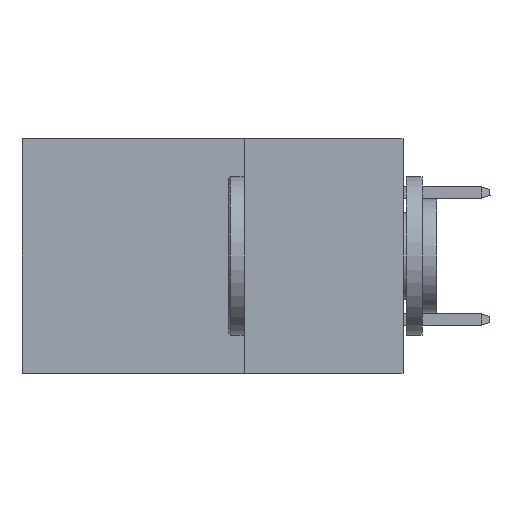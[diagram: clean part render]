
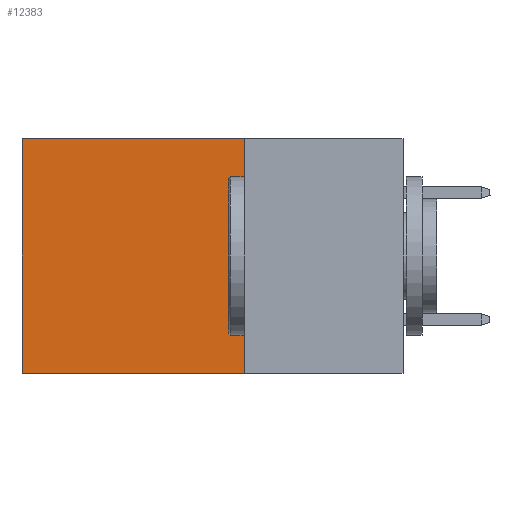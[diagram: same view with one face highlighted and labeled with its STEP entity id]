
A CAD part, left-side view. The second image highlights one B-rep face of the part: STEP entity #12383.
In plain terms, the highlighted planar face has unit normal (-1, 0, 0).
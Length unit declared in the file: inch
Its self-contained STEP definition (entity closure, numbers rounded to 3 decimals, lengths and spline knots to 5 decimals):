
#3955 = VERTEX_POINT ( 'NONE', #8767 ) ;
#5047 = DIRECTION ( 'NONE',  ( 0., 1., 0. ) ) ;
#6533 = ORIENTED_EDGE ( 'NONE', *, *, #20323, .T. ) ;
#8109 = DIRECTION ( 'NONE',  ( 0., 1., 0. ) ) ;
#8767 = CARTESIAN_POINT ( 'NONE',  ( 0.2875, 0.25, -0.37 ) ) ;
#9014 = CARTESIAN_POINT ( 'NONE',  ( 0.2875, 0.25, 0. ) ) ;
#9194 = ORIENTED_EDGE ( 'NONE', *, *, #35555, .F. ) ;
#11284 = CARTESIAN_POINT ( 'NONE',  ( 0.2875, 0.25, 0. ) ) ;
#11391 = VERTEX_POINT ( 'NONE', #26016 ) ;
#12294 = DIRECTION ( 'NONE',  ( 0., 0., -1. ) ) ;
#12383 = ADVANCED_FACE ( 'NONE', ( #35965 ), #30288, .F. ) ;
#14597 = CARTESIAN_POINT ( 'NONE',  ( 0.2875, 0.25, 0. ) ) ;
#16473 = EDGE_CURVE ( 'NONE', #29625, #3955, #30131, .T. ) ;
#16636 = CARTESIAN_POINT ( 'NONE',  ( 0.2875, 0.25, -0.37 ) ) ;
#20323 = EDGE_CURVE ( 'NONE', #29625, #11391, #28796, .T. ) ;
#21387 = CARTESIAN_POINT ( 'NONE',  ( 0.2875, 0.25, 0. ) ) ;
#22755 = EDGE_CURVE ( 'NONE', #11391, #36157, #24646, .T. ) ;
#23170 = LINE ( 'NONE', #16636, #23257 ) ;
#23257 = VECTOR ( 'NONE', #5047, 39.37008 ) ;
#24646 = LINE ( 'NONE', #25030, #35932 ) ;
#25019 = CARTESIAN_POINT ( 'NONE',  ( 0.2875, 0.6, -0.37 ) ) ;
#25030 = CARTESIAN_POINT ( 'NONE',  ( 0.2875, 0.6, 0. ) ) ;
#26016 = CARTESIAN_POINT ( 'NONE',  ( 0.2875, 0.6, 0. ) ) ;
#28796 = LINE ( 'NONE', #14597, #28913 ) ;
#28913 = VECTOR ( 'NONE', #8109, 39.37008 ) ;
#29472 = ORIENTED_EDGE ( 'NONE', *, *, #16473, .F. ) ;
#29625 = VERTEX_POINT ( 'NONE', #11284 ) ;
#30131 = LINE ( 'NONE', #9014, #38879 ) ;
#30288 = PLANE ( 'NONE',  #30490 ) ;
#30490 = AXIS2_PLACEMENT_3D ( 'NONE', #21387, #30657, #12294 ) ;
#30657 = DIRECTION ( 'NONE',  ( 1., 0., 0. ) ) ;
#32648 = EDGE_LOOP ( 'NONE', ( #38273, #9194, #29472, #6533 ) ) ;
#33235 = DIRECTION ( 'NONE',  ( 0., 0., -1. ) ) ;
#34449 = DIRECTION ( 'NONE',  ( 0., 0., -1. ) ) ;
#35555 = EDGE_CURVE ( 'NONE', #3955, #36157, #23170, .T. ) ;
#35932 = VECTOR ( 'NONE', #34449, 39.37008 ) ;
#35965 = FACE_OUTER_BOUND ( 'NONE', #32648, .T. ) ;
#36157 = VERTEX_POINT ( 'NONE', #25019 ) ;
#38273 = ORIENTED_EDGE ( 'NONE', *, *, #22755, .T. ) ;
#38879 = VECTOR ( 'NONE', #33235, 39.37008 ) ;
